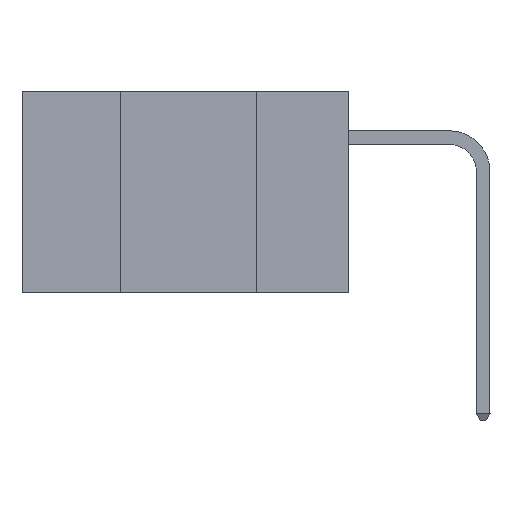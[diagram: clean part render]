
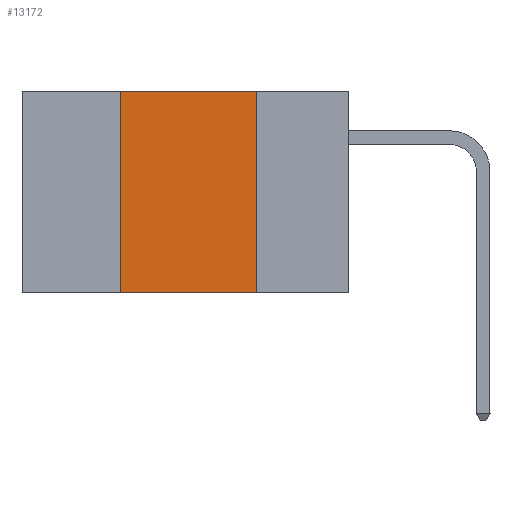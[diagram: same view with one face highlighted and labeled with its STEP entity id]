
A CAD part, left-side view. The second image highlights one B-rep face of the part: STEP entity #13172.
In plain terms, the highlighted planar face has unit normal (-1, 0, 0).
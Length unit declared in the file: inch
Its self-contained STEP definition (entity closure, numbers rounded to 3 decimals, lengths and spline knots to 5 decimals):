
#1223 = VERTEX_POINT ( 'NONE', #16342 ) ;
#2124 = DIRECTION ( 'NONE',  ( 0., -1., 0. ) ) ;
#2139 = EDGE_CURVE ( 'NONE', #1223, #4231, #3740, .T. ) ;
#2164 = ORIENTED_EDGE ( 'NONE', *, *, #8074, .F. ) ;
#2362 = ORIENTED_EDGE ( 'NONE', *, *, #4108, .F. ) ;
#3307 = VECTOR ( 'NONE', #2124, 39.37008 ) ;
#3740 = LINE ( 'NONE', #15298, #3307 ) ;
#4108 = EDGE_CURVE ( 'NONE', #4231, #5048, #14680, .T. ) ;
#4231 = VERTEX_POINT ( 'NONE', #7427 ) ;
#4465 = DIRECTION ( 'NONE',  ( 0., 0., -1. ) ) ;
#4732 = CARTESIAN_POINT ( 'NONE',  ( 0., 0.17, -0.37 ) ) ;
#4778 = EDGE_LOOP ( 'NONE', ( #2362, #7073, #2164, #13767 ) ) ;
#4801 = CARTESIAN_POINT ( 'NONE',  ( 0., 0.6, -0.37 ) ) ;
#5048 = VERTEX_POINT ( 'NONE', #4732 ) ;
#5252 = AXIS2_PLACEMENT_3D ( 'NONE', #16084, #10979, #11073 ) ;
#5663 = CARTESIAN_POINT ( 'NONE',  ( 0., 0.42, -0.37 ) ) ;
#6314 = LINE ( 'NONE', #4801, #15349 ) ;
#6534 = DIRECTION ( 'NONE',  ( 0., 0., 1. ) ) ;
#7073 = ORIENTED_EDGE ( 'NONE', *, *, #2139, .F. ) ;
#7427 = CARTESIAN_POINT ( 'NONE',  ( 0., 0.17, 0. ) ) ;
#8074 = EDGE_CURVE ( 'NONE', #8153, #1223, #13011, .T. ) ;
#8153 = VERTEX_POINT ( 'NONE', #5663 ) ;
#8352 = PLANE ( 'NONE',  #5252 ) ;
#8466 = CARTESIAN_POINT ( 'NONE',  ( 0., 0.17, 0. ) ) ;
#10979 = DIRECTION ( 'NONE',  ( 1., 0., 0. ) ) ;
#11073 = DIRECTION ( 'NONE',  ( 0., 0., -1. ) ) ;
#13011 = LINE ( 'NONE', #13160, #14044 ) ;
#13160 = CARTESIAN_POINT ( 'NONE',  ( 0., 0.42, 0. ) ) ;
#13172 = ADVANCED_FACE ( 'NONE', ( #14906 ), #8352, .F. ) ;
#13767 = ORIENTED_EDGE ( 'NONE', *, *, #15758, .T. ) ;
#14044 = VECTOR ( 'NONE', #6534, 39.37008 ) ;
#14495 = VECTOR ( 'NONE', #4465, 39.37008 ) ;
#14680 = LINE ( 'NONE', #8466, #14495 ) ;
#14906 = FACE_OUTER_BOUND ( 'NONE', #4778, .T. ) ;
#15298 = CARTESIAN_POINT ( 'NONE',  ( 0., 0.6, 0. ) ) ;
#15349 = VECTOR ( 'NONE', #16548, 39.37008 ) ;
#15758 = EDGE_CURVE ( 'NONE', #8153, #5048, #6314, .T. ) ;
#16084 = CARTESIAN_POINT ( 'NONE',  ( 0., 0.6, 0. ) ) ;
#16342 = CARTESIAN_POINT ( 'NONE',  ( 0., 0.42, 0. ) ) ;
#16548 = DIRECTION ( 'NONE',  ( 0., -1., 0. ) ) ;
